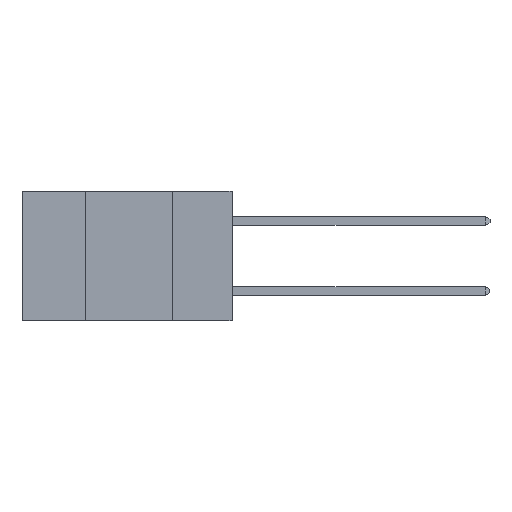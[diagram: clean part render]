
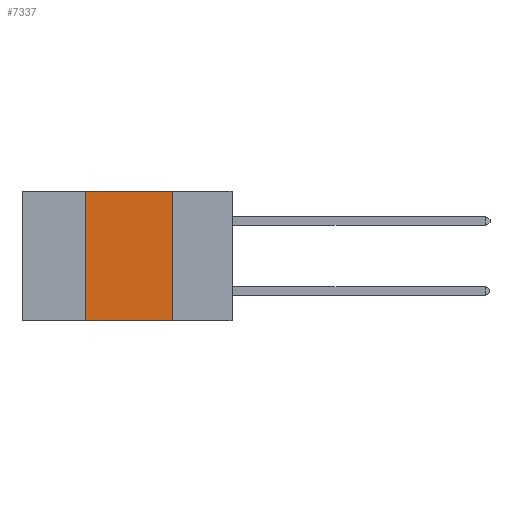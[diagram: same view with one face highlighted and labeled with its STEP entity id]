
A CAD part, left-side view. The second image highlights one B-rep face of the part: STEP entity #7337.
In plain terms, the highlighted planar face has unit normal (-1, 0, 0).
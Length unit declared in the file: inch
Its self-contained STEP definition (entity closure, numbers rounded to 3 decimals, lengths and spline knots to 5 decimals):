
#756 = AXIS2_PLACEMENT_3D ( 'NONE', #16766, #18362, #8577 ) ;
#1157 = FACE_OUTER_BOUND ( 'NONE', #16512, .T. ) ;
#2080 = CARTESIAN_POINT ( 'NONE',  ( 0., 0.17, 0. ) ) ;
#4068 = CARTESIAN_POINT ( 'NONE',  ( 0., 0.6, 0. ) ) ;
#4276 = CARTESIAN_POINT ( 'NONE',  ( 0., 0.42, -0.37 ) ) ;
#5247 = PLANE ( 'NONE',  #756 ) ;
#5416 = VECTOR ( 'NONE', #18473, 39.37008 ) ;
#6016 = LINE ( 'NONE', #16229, #13687 ) ;
#7337 = ADVANCED_FACE ( 'NONE', ( #1157 ), #5247, .F. ) ;
#8577 = DIRECTION ( 'NONE',  ( 0., 0., -1. ) ) ;
#9689 = EDGE_CURVE ( 'NONE', #16343, #19355, #6016, .T. ) ;
#9696 = DIRECTION ( 'NONE',  ( 0., 0., 1. ) ) ;
#9697 = DIRECTION ( 'NONE',  ( 0., -1., 0. ) ) ;
#10140 = ORIENTED_EDGE ( 'NONE', *, *, #19442, .F. ) ;
#10779 = LINE ( 'NONE', #17769, #18436 ) ;
#11515 = ORIENTED_EDGE ( 'NONE', *, *, #18338, .F. ) ;
#11851 = CARTESIAN_POINT ( 'NONE',  ( 0., 0.17, -0.37 ) ) ;
#12912 = EDGE_CURVE ( 'NONE', #16343, #13650, #10779, .T. ) ;
#13650 = VERTEX_POINT ( 'NONE', #16413 ) ;
#13687 = VECTOR ( 'NONE', #9697, 39.37008 ) ;
#14138 = LINE ( 'NONE', #2080, #5416 ) ;
#14347 = ORIENTED_EDGE ( 'NONE', *, *, #12912, .F. ) ;
#14927 = ORIENTED_EDGE ( 'NONE', *, *, #9689, .T. ) ;
#15207 = VERTEX_POINT ( 'NONE', #16247 ) ;
#16229 = CARTESIAN_POINT ( 'NONE',  ( 0., 0.6, -0.37 ) ) ;
#16247 = CARTESIAN_POINT ( 'NONE',  ( 0., 0.17, 0. ) ) ;
#16343 = VERTEX_POINT ( 'NONE', #4276 ) ;
#16413 = CARTESIAN_POINT ( 'NONE',  ( 0., 0.42, 0. ) ) ;
#16512 = EDGE_LOOP ( 'NONE', ( #10140, #11515, #14347, #14927 ) ) ;
#16766 = CARTESIAN_POINT ( 'NONE',  ( 0., 0.6, 0. ) ) ;
#17769 = CARTESIAN_POINT ( 'NONE',  ( 0., 0.42, 0. ) ) ;
#17961 = LINE ( 'NONE', #4068, #20655 ) ;
#18338 = EDGE_CURVE ( 'NONE', #13650, #15207, #17961, .T. ) ;
#18362 = DIRECTION ( 'NONE',  ( 1., 0., 0. ) ) ;
#18436 = VECTOR ( 'NONE', #9696, 39.37008 ) ;
#18473 = DIRECTION ( 'NONE',  ( 0., 0., -1. ) ) ;
#18774 = DIRECTION ( 'NONE',  ( 0., -1., 0. ) ) ;
#19355 = VERTEX_POINT ( 'NONE', #11851 ) ;
#19442 = EDGE_CURVE ( 'NONE', #15207, #19355, #14138, .T. ) ;
#20655 = VECTOR ( 'NONE', #18774, 39.37008 ) ;
